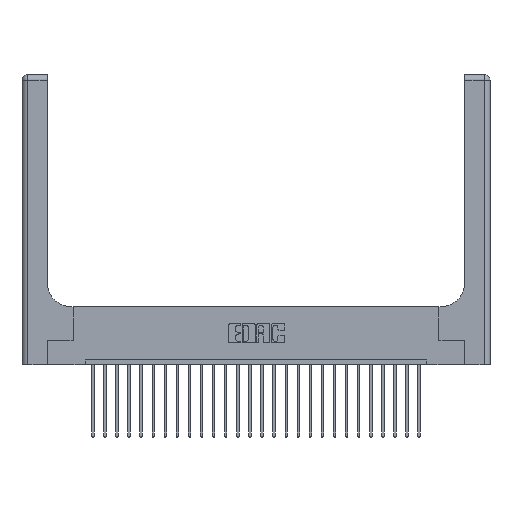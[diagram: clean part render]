
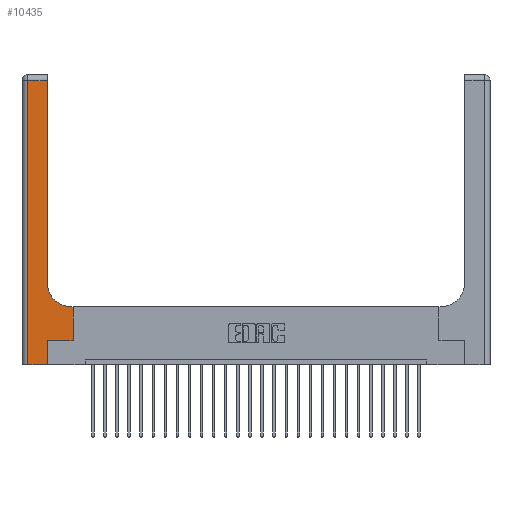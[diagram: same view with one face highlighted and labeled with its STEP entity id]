
A CAD part, top view. The second image highlights one B-rep face of the part: STEP entity #10435.
In plain terms, the highlighted planar face has unit normal (0, 0, 1).
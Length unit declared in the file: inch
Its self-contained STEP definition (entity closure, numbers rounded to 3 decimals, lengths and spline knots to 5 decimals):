
#216 = DIRECTION ( 'NONE',  ( -1., 0., 0. ) ) ;
#475 = DIRECTION ( 'NONE',  ( -1., 0., 0. ) ) ;
#500 = EDGE_CURVE ( 'NONE', #12737, #5828, #18596, .T. ) ;
#1107 = VECTOR ( 'NONE', #6131, 39.37008 ) ;
#1406 = VERTEX_POINT ( 'NONE', #5106 ) ;
#1806 = CARTESIAN_POINT ( 'NONE',  ( 0.26, 3., 0.37 ) ) ;
#2215 = LINE ( 'NONE', #6374, #1107 ) ;
#2332 = ORIENTED_EDGE ( 'NONE', *, *, #23018, .T. ) ;
#2829 = LINE ( 'NONE', #10529, #19118 ) ;
#3466 = VECTOR ( 'NONE', #216, 39.37008 ) ;
#3587 = CARTESIAN_POINT ( 'NONE',  ( 0.265, 0.25, 0.37 ) ) ;
#3647 = EDGE_CURVE ( 'NONE', #15089, #13059, #2829, .T. ) ;
#4709 = ORIENTED_EDGE ( 'NONE', *, *, #23543, .T. ) ;
#4933 = DIRECTION ( 'NONE',  ( 1., 0., 0. ) ) ;
#4965 = LINE ( 'NONE', #1806, #7220 ) ;
#5106 = CARTESIAN_POINT ( 'NONE',  ( 0.528, 0.6, 0.37 ) ) ;
#5201 = EDGE_CURVE ( 'NONE', #18721, #11653, #19116, .T. ) ;
#5761 = CARTESIAN_POINT ( 'NONE',  ( 0.06, 3., 0.37 ) ) ;
#5828 = VERTEX_POINT ( 'NONE', #9196 ) ;
#5879 = CARTESIAN_POINT ( 'NONE',  ( 0., 2.94, 0.37 ) ) ;
#6131 = DIRECTION ( 'NONE',  ( 0., 1., 0. ) ) ;
#6374 = CARTESIAN_POINT ( 'NONE',  ( 0.528, 0.25, 0.37 ) ) ;
#6494 = EDGE_CURVE ( 'NONE', #13489, #1406, #2215, .T. ) ;
#6679 = CARTESIAN_POINT ( 'NONE',  ( 0.265, 0.25, 0.37 ) ) ;
#6697 = DIRECTION ( 'NONE',  ( 0., 0., -1. ) ) ;
#7161 = ORIENTED_EDGE ( 'NONE', *, *, #17496, .T. ) ;
#7220 = VECTOR ( 'NONE', #24865, 39.37008 ) ;
#7556 = CARTESIAN_POINT ( 'NONE',  ( 0., 3., 0.37 ) ) ;
#9036 = CARTESIAN_POINT ( 'NONE',  ( 0.265, 0., 0.37 ) ) ;
#9196 = CARTESIAN_POINT ( 'NONE',  ( 0.26, 0.85, 0.37 ) ) ;
#9572 = FACE_OUTER_BOUND ( 'NONE', #10611, .T. ) ;
#9618 = CARTESIAN_POINT ( 'NONE',  ( 0.265, 0., 0.37 ) ) ;
#9638 = AXIS2_PLACEMENT_3D ( 'NONE', #7556, #13360, #17115 ) ;
#10043 = CARTESIAN_POINT ( 'NONE',  ( 0.26, 0.6, 0.37 ) ) ;
#10435 = ADVANCED_FACE ( 'NONE', ( #9572 ), #23189, .F. ) ;
#10509 = ORIENTED_EDGE ( 'NONE', *, *, #5201, .T. ) ;
#10529 = CARTESIAN_POINT ( 'NONE',  ( 0., 0., 0.37 ) ) ;
#10541 = AXIS2_PLACEMENT_3D ( 'NONE', #23970, #6697, #4933 ) ;
#10611 = EDGE_LOOP ( 'NONE', ( #4709, #10509, #20855, #12728, #22377, #7161, #19332, #2332, #20527 ) ) ;
#11585 = CARTESIAN_POINT ( 'NONE',  ( 0.51, 0.6, 0.37 ) ) ;
#11653 = VERTEX_POINT ( 'NONE', #21911 ) ;
#11995 = CARTESIAN_POINT ( 'NONE',  ( 0.06, 0., 0.37 ) ) ;
#12728 = ORIENTED_EDGE ( 'NONE', *, *, #3647, .T. ) ;
#12737 = VERTEX_POINT ( 'NONE', #11585 ) ;
#13059 = VERTEX_POINT ( 'NONE', #9036 ) ;
#13196 = LINE ( 'NONE', #5761, #21653 ) ;
#13360 = DIRECTION ( 'NONE',  ( 0., 0., -1. ) ) ;
#13489 = VERTEX_POINT ( 'NONE', #22507 ) ;
#13651 = CARTESIAN_POINT ( 'NONE',  ( 0.26, 2.94, 0.37 ) ) ;
#13824 = VECTOR ( 'NONE', #23252, 39.37008 ) ;
#14429 = DIRECTION ( 'NONE',  ( 1., 0., 0. ) ) ;
#15089 = VERTEX_POINT ( 'NONE', #11995 ) ;
#15097 = EDGE_CURVE ( 'NONE', #13059, #21511, #19203, .T. ) ;
#17022 = VECTOR ( 'NONE', #23858, 39.37008 ) ;
#17115 = DIRECTION ( 'NONE',  ( -1., 0., 0. ) ) ;
#17496 = EDGE_CURVE ( 'NONE', #21511, #13489, #20865, .T. ) ;
#18596 = CIRCLE ( 'NONE', #10541, 0.25 ) ;
#18721 = VERTEX_POINT ( 'NONE', #13651 ) ;
#19116 = LINE ( 'NONE', #5879, #3466 ) ;
#19118 = VECTOR ( 'NONE', #14429, 39.37008 ) ;
#19203 = LINE ( 'NONE', #9618, #17022 ) ;
#19332 = ORIENTED_EDGE ( 'NONE', *, *, #6494, .T. ) ;
#20245 = LINE ( 'NONE', #10043, #22908 ) ;
#20527 = ORIENTED_EDGE ( 'NONE', *, *, #500, .T. ) ;
#20855 = ORIENTED_EDGE ( 'NONE', *, *, #22028, .T. ) ;
#20865 = LINE ( 'NONE', #3587, #13824 ) ;
#21511 = VERTEX_POINT ( 'NONE', #6679 ) ;
#21653 = VECTOR ( 'NONE', #22911, 39.37008 ) ;
#21911 = CARTESIAN_POINT ( 'NONE',  ( 0.06, 2.94, 0.37 ) ) ;
#22028 = EDGE_CURVE ( 'NONE', #11653, #15089, #13196, .T. ) ;
#22377 = ORIENTED_EDGE ( 'NONE', *, *, #15097, .T. ) ;
#22507 = CARTESIAN_POINT ( 'NONE',  ( 0.528, 0.25, 0.37 ) ) ;
#22908 = VECTOR ( 'NONE', #475, 39.37008 ) ;
#22911 = DIRECTION ( 'NONE',  ( 0., -1., 0. ) ) ;
#23018 = EDGE_CURVE ( 'NONE', #1406, #12737, #20245, .T. ) ;
#23189 = PLANE ( 'NONE',  #9638 ) ;
#23252 = DIRECTION ( 'NONE',  ( 1., 0., 0. ) ) ;
#23543 = EDGE_CURVE ( 'NONE', #5828, #18721, #4965, .T. ) ;
#23858 = DIRECTION ( 'NONE',  ( 0., 1., 0. ) ) ;
#23970 = CARTESIAN_POINT ( 'NONE',  ( 0.51, 0.85, 0.37 ) ) ;
#24865 = DIRECTION ( 'NONE',  ( 0., 1., 0. ) ) ;
